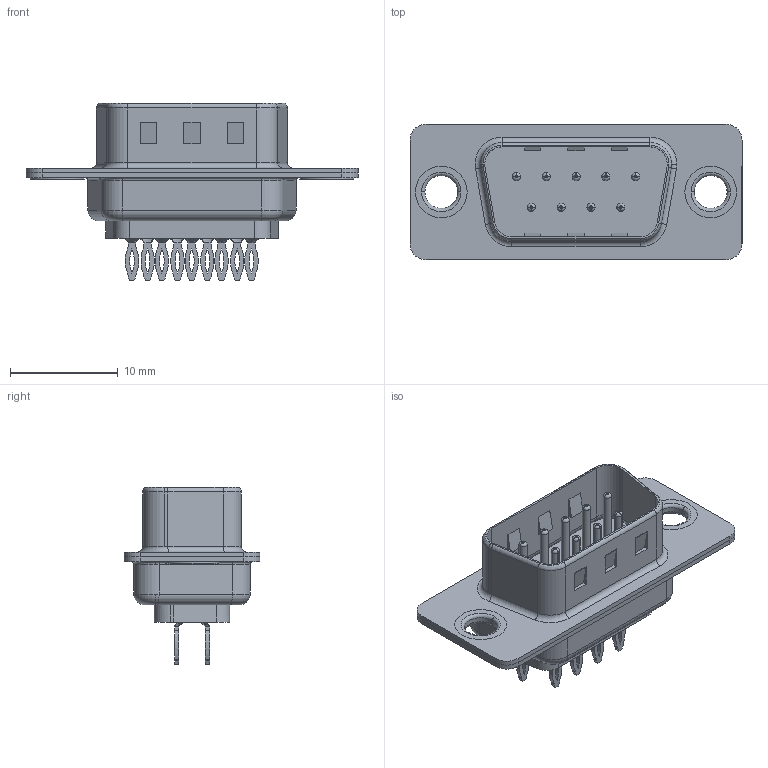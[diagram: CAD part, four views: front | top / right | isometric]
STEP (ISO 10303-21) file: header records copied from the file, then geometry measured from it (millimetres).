
FILE_DESCRIPTION (( 'STEP AP203' ), '1' );
FILE_NAME ('627-009-326-261.STEP', '2020-07-14T02:33:15', ( '' ), ( '' ), 'SwSTEP 2.0', 'SolidWorks 2020', '' );
FILE_SCHEMA (( 'CONFIG_CONTROL_DESIGN' ));
Length unit declared in the file: millimetre
Products named in the file (7): 627 Housing_09 LP; 627-009-326-261; 627 Thru Hole Rivet; 627 Shell Rear_09 Contacts; 627 Contact Row 1_26L; 627 Contact Row 2_26L; 627 Shell Front_09 Contacts
Assembly tree (14 placements, depth 2):
  627-009-326-261
    627 Housing_09 LP
    627 Shell Front_09 Contacts
    627 Shell Rear_09 Contacts
    627 Contact Row 1_26L  x5
    627 Contact Row 2_26L  x4
    627 Thru Hole Rivet  x2
Bounding box: 30.8 x 12.6 x 16.45 mm (x, y, z)
Volume: 1233.8 mm3; surface area: 3760.7 mm2
Topology: 14 solids, 14 shells, 962 faces, 2403 edges, 1498 vertices
Faces by surface type: cylinder 392, plane 287, torus 247, bspline 36
Entity records: 15149 total; most frequent: CARTESIAN_POINT 2674, DIRECTION 2625, ORIENTED_EDGE 2290, EDGE_CURVE 1145, AXIS2_PLACEMENT_3D 1044, VERTEX_POINT 718, CIRCLE 569, EDGE_LOOP 541
